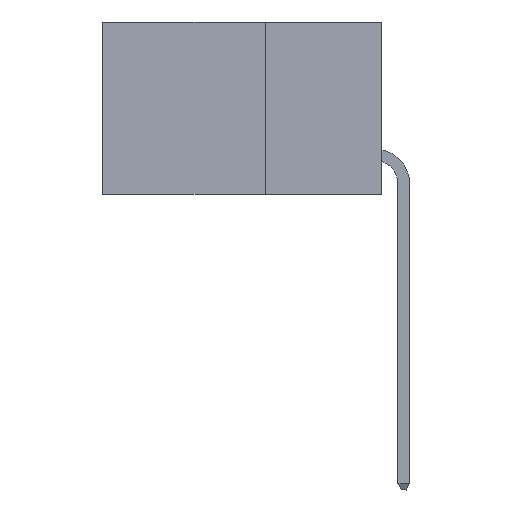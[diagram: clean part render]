
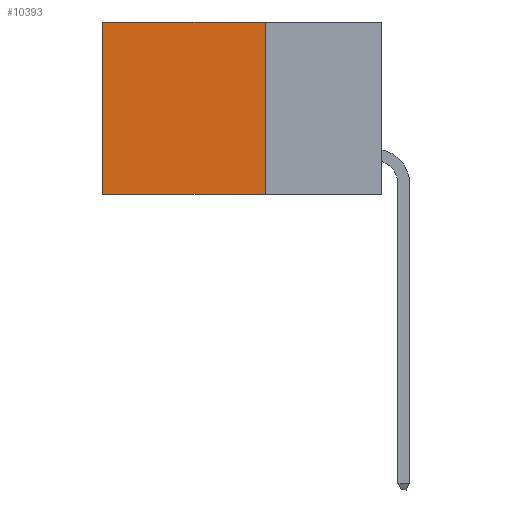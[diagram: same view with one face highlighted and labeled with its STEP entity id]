
A CAD part, left-side view. The second image highlights one B-rep face of the part: STEP entity #10393.
In plain terms, the highlighted planar face has unit normal (-1, 0, 0).
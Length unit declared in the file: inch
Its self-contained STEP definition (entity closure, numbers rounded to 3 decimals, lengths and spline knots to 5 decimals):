
#324 = ORIENTED_EDGE ( 'NONE', *, *, #5499, .F. ) ;
#866 = EDGE_LOOP ( 'NONE', ( #1908, #324, #10141, #12199 ) ) ;
#1379 = EDGE_CURVE ( 'NONE', #13003, #14727, #10701, .T. ) ;
#1908 = ORIENTED_EDGE ( 'NONE', *, *, #4835, .T. ) ;
#1985 = EDGE_CURVE ( 'NONE', #13003, #7469, #2344, .T. ) ;
#2344 = LINE ( 'NONE', #15433, #14149 ) ;
#2438 = DIRECTION ( 'NONE',  ( 0., 0., -1. ) ) ;
#2463 = DIRECTION ( 'NONE',  ( 1., 0., 0. ) ) ;
#2475 = CARTESIAN_POINT ( 'NONE',  ( 0.2875, 0.25, -0.37 ) ) ;
#2736 = PLANE ( 'NONE',  #15068 ) ;
#3415 = VECTOR ( 'NONE', #13806, 39.37008 ) ;
#4835 = EDGE_CURVE ( 'NONE', #14727, #9338, #9445, .T. ) ;
#4911 = DIRECTION ( 'NONE',  ( 0., 1., 0. ) ) ;
#5479 = CARTESIAN_POINT ( 'NONE',  ( 0.2875, 0.6, 0. ) ) ;
#5499 = EDGE_CURVE ( 'NONE', #7469, #9338, #18098, .T. ) ;
#6177 = VECTOR ( 'NONE', #6724, 39.37008 ) ;
#6360 = CARTESIAN_POINT ( 'NONE',  ( 0.2875, 0.25, -0.37 ) ) ;
#6724 = DIRECTION ( 'NONE',  ( 0., 0., -1. ) ) ;
#7469 = VERTEX_POINT ( 'NONE', #2475 ) ;
#9338 = VERTEX_POINT ( 'NONE', #17232 ) ;
#9445 = LINE ( 'NONE', #16801, #6177 ) ;
#9825 = FACE_OUTER_BOUND ( 'NONE', #866, .T. ) ;
#10141 = ORIENTED_EDGE ( 'NONE', *, *, #1985, .F. ) ;
#10393 = ADVANCED_FACE ( 'NONE', ( #9825 ), #2736, .F. ) ;
#10701 = LINE ( 'NONE', #15160, #3415 ) ;
#12199 = ORIENTED_EDGE ( 'NONE', *, *, #1379, .T. ) ;
#13003 = VERTEX_POINT ( 'NONE', #14411 ) ;
#13806 = DIRECTION ( 'NONE',  ( 0., 1., 0. ) ) ;
#14149 = VECTOR ( 'NONE', #2438, 39.37008 ) ;
#14411 = CARTESIAN_POINT ( 'NONE',  ( 0.2875, 0.25, 0. ) ) ;
#14727 = VERTEX_POINT ( 'NONE', #5479 ) ;
#15068 = AXIS2_PLACEMENT_3D ( 'NONE', #15740, #2463, #18743 ) ;
#15160 = CARTESIAN_POINT ( 'NONE',  ( 0.2875, 0.25, 0. ) ) ;
#15433 = CARTESIAN_POINT ( 'NONE',  ( 0.2875, 0.25, 0. ) ) ;
#15740 = CARTESIAN_POINT ( 'NONE',  ( 0.2875, 0.25, 0. ) ) ;
#16801 = CARTESIAN_POINT ( 'NONE',  ( 0.2875, 0.6, 0. ) ) ;
#16840 = VECTOR ( 'NONE', #4911, 39.37008 ) ;
#17232 = CARTESIAN_POINT ( 'NONE',  ( 0.2875, 0.6, -0.37 ) ) ;
#18098 = LINE ( 'NONE', #6360, #16840 ) ;
#18743 = DIRECTION ( 'NONE',  ( 0., 0., -1. ) ) ;
